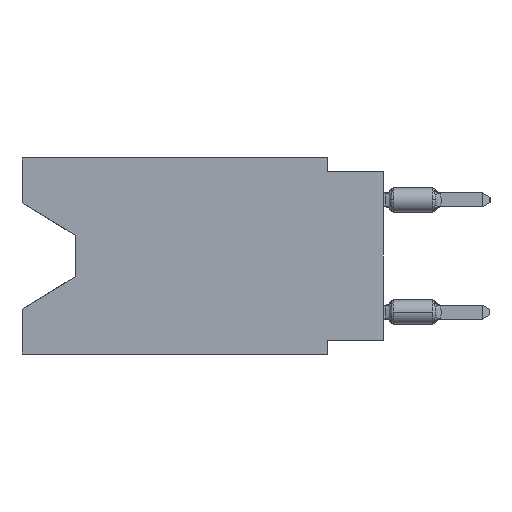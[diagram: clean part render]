
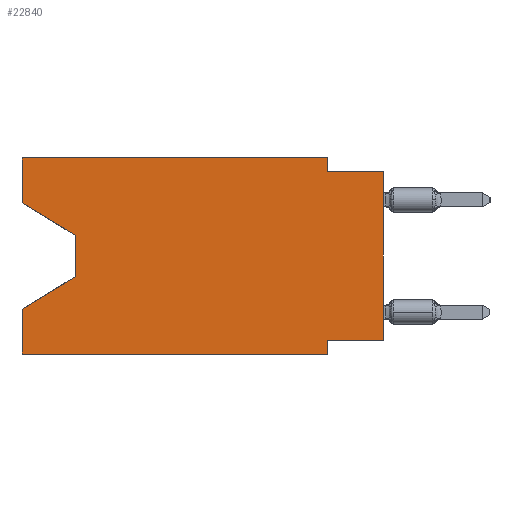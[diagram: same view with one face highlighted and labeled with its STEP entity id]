
A CAD part, left-side view. The second image highlights one B-rep face of the part: STEP entity #22840.
In plain terms, the highlighted planar face has unit normal (-1, 0, 0).
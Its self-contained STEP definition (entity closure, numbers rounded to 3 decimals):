
#190 = VERTEX_POINT ( 'NONE', #10890 ) ;
#904 = EDGE_LOOP ( 'NONE', ( #8589, #33899, #34542, #11193, #36317, #41280, #9095, #8226, #21461, #13554, #28977, #25182 ) ) ;
#2224 = LINE ( 'NONE', #29516, #17012 ) ;
#2622 = CARTESIAN_POINT ( 'NONE',  ( 0., 16.383, -2.038 ) ) ;
#5558 = EDGE_CURVE ( 'NONE', #40403, #23073, #16838, .T. ) ;
#5756 = CARTESIAN_POINT ( 'NONE',  ( 0., 16.383, -2.038 ) ) ;
#6208 = CARTESIAN_POINT ( 'NONE',  ( 0., 13.97, -5.385 ) ) ;
#6732 = CARTESIAN_POINT ( 'NONE',  ( 0., 13.97, -3.505 ) ) ;
#7610 = DIRECTION ( 'NONE',  ( 0., -1., 0. ) ) ;
#8206 = AXIS2_PLACEMENT_3D ( 'NONE', #37089, #36657, #29904 ) ;
#8226 = ORIENTED_EDGE ( 'NONE', *, *, #33989, .T. ) ;
#8589 = ORIENTED_EDGE ( 'NONE', *, *, #15736, .T. ) ;
#9095 = ORIENTED_EDGE ( 'NONE', *, *, #40701, .F. ) ;
#9105 = CARTESIAN_POINT ( 'NONE',  ( 0., 16.383, 0. ) ) ;
#9163 = CARTESIAN_POINT ( 'NONE',  ( 0., 2.54, -0.635 ) ) ;
#9471 = DIRECTION ( 'NONE',  ( 0., 0., 1. ) ) ;
#9561 = PLANE ( 'NONE',  #8206 ) ;
#9718 = VERTEX_POINT ( 'NONE', #30512 ) ;
#10890 = CARTESIAN_POINT ( 'NONE',  ( 0., 0., -8.255 ) ) ;
#11113 = LINE ( 'NONE', #13944, #34007 ) ;
#11193 = ORIENTED_EDGE ( 'NONE', *, *, #12792, .F. ) ;
#11499 = VECTOR ( 'NONE', #32435, 1000. ) ;
#12535 = LINE ( 'NONE', #39009, #38154 ) ;
#12792 = EDGE_CURVE ( 'NONE', #14418, #38018, #12535, .T. ) ;
#13004 = DIRECTION ( 'NONE',  ( 0., -1., 0. ) ) ;
#13524 = CARTESIAN_POINT ( 'NONE',  ( 0., 16.383, 0. ) ) ;
#13554 = ORIENTED_EDGE ( 'NONE', *, *, #5558, .F. ) ;
#13653 = EDGE_CURVE ( 'NONE', #9718, #40403, #20005, .T. ) ;
#13944 = CARTESIAN_POINT ( 'NONE',  ( 0., 13.97, -3.505 ) ) ;
#14418 = VERTEX_POINT ( 'NONE', #29110 ) ;
#14885 = EDGE_CURVE ( 'NONE', #36836, #35795, #22056, .T. ) ;
#14917 = VERTEX_POINT ( 'NONE', #2622 ) ;
#15736 = EDGE_CURVE ( 'NONE', #14917, #36433, #35714, .T. ) ;
#16089 = CARTESIAN_POINT ( 'NONE',  ( 0., 2.54, 0. ) ) ;
#16434 = CARTESIAN_POINT ( 'NONE',  ( 0., 2.54, -8.89 ) ) ;
#16674 = DIRECTION ( 'NONE',  ( 0., 0.855, -0.519 ) ) ;
#16838 = LINE ( 'NONE', #33683, #41931 ) ;
#17012 = VECTOR ( 'NONE', #29310, 1000. ) ;
#18340 = VECTOR ( 'NONE', #13004, 1000. ) ;
#18405 = EDGE_CURVE ( 'NONE', #39146, #38018, #36369, .T. ) ;
#19142 = CARTESIAN_POINT ( 'NONE',  ( 0., 16.383, -8.89 ) ) ;
#19164 = DIRECTION ( 'NONE',  ( 0., -1., 0. ) ) ;
#19407 = FACE_OUTER_BOUND ( 'NONE', #904, .T. ) ;
#20005 = LINE ( 'NONE', #9105, #21769 ) ;
#20494 = EDGE_CURVE ( 'NONE', #14418, #35795, #22855, .T. ) ;
#20990 = DIRECTION ( 'NONE',  ( 0., 0., -1. ) ) ;
#21461 = ORIENTED_EDGE ( 'NONE', *, *, #40191, .F. ) ;
#21604 = CARTESIAN_POINT ( 'NONE',  ( 0., 0., -0.635 ) ) ;
#21769 = VECTOR ( 'NONE', #19164, 1000. ) ;
#22056 = LINE ( 'NONE', #42412, #29543 ) ;
#22391 = DIRECTION ( 'NONE',  ( 0., 1., 0. ) ) ;
#22840 = ADVANCED_FACE ( 'NONE', ( #19407 ), #9561, .F. ) ;
#22855 = LINE ( 'NONE', #19142, #18340 ) ;
#23073 = VERTEX_POINT ( 'NONE', #9163 ) ;
#23202 = VECTOR ( 'NONE', #16674, 1000. ) ;
#23370 = LINE ( 'NONE', #13524, #30508 ) ;
#23520 = VECTOR ( 'NONE', #22391, 1000. ) ;
#24440 = DIRECTION ( 'NONE',  ( 0., 0., -1. ) ) ;
#25182 = ORIENTED_EDGE ( 'NONE', *, *, #32369, .F. ) ;
#25457 = CARTESIAN_POINT ( 'NONE',  ( 0., 0., -8.255 ) ) ;
#26019 = DIRECTION ( 'NONE',  ( 0., 0., 1. ) ) ;
#27126 = VERTEX_POINT ( 'NONE', #21604 ) ;
#28142 = LINE ( 'NONE', #41479, #33943 ) ;
#28838 = DIRECTION ( 'NONE',  ( 0., 0., -1. ) ) ;
#28949 = LINE ( 'NONE', #25457, #23520 ) ;
#28977 = ORIENTED_EDGE ( 'NONE', *, *, #13653, .F. ) ;
#29110 = CARTESIAN_POINT ( 'NONE',  ( 0., 16.383, -8.89 ) ) ;
#29310 = DIRECTION ( 'NONE',  ( 0., 0., 1. ) ) ;
#29516 = CARTESIAN_POINT ( 'NONE',  ( 0., 0., 0. ) ) ;
#29543 = VECTOR ( 'NONE', #28838, 1000. ) ;
#29904 = DIRECTION ( 'NONE',  ( 0., 0., -1. ) ) ;
#30508 = VECTOR ( 'NONE', #26019, 1000. ) ;
#30512 = CARTESIAN_POINT ( 'NONE',  ( 0., 16.383, 0. ) ) ;
#32369 = EDGE_CURVE ( 'NONE', #14917, #9718, #23370, .T. ) ;
#32435 = DIRECTION ( 'NONE',  ( 0., -0.855, -0.519 ) ) ;
#33683 = CARTESIAN_POINT ( 'NONE',  ( 0., 2.54, 0. ) ) ;
#33899 = ORIENTED_EDGE ( 'NONE', *, *, #43044, .T. ) ;
#33943 = VECTOR ( 'NONE', #7610, 1000. ) ;
#33989 = EDGE_CURVE ( 'NONE', #190, #27126, #2224, .T. ) ;
#34007 = VECTOR ( 'NONE', #24440, 1000. ) ;
#34542 = ORIENTED_EDGE ( 'NONE', *, *, #18405, .T. ) ;
#35714 = LINE ( 'NONE', #5756, #11499 ) ;
#35795 = VERTEX_POINT ( 'NONE', #16434 ) ;
#36317 = ORIENTED_EDGE ( 'NONE', *, *, #20494, .T. ) ;
#36369 = LINE ( 'NONE', #6208, #23202 ) ;
#36433 = VERTEX_POINT ( 'NONE', #6732 ) ;
#36657 = DIRECTION ( 'NONE',  ( 1., 0., 0. ) ) ;
#36836 = VERTEX_POINT ( 'NONE', #38417 ) ;
#37089 = CARTESIAN_POINT ( 'NONE',  ( 0., 16.383, 0. ) ) ;
#38018 = VERTEX_POINT ( 'NONE', #42358 ) ;
#38154 = VECTOR ( 'NONE', #9471, 1000. ) ;
#38417 = CARTESIAN_POINT ( 'NONE',  ( 0., 2.54, -8.255 ) ) ;
#39009 = CARTESIAN_POINT ( 'NONE',  ( 0., 16.383, 0. ) ) ;
#39146 = VERTEX_POINT ( 'NONE', #39270 ) ;
#39270 = CARTESIAN_POINT ( 'NONE',  ( 0., 13.97, -5.385 ) ) ;
#40191 = EDGE_CURVE ( 'NONE', #23073, #27126, #28142, .T. ) ;
#40403 = VERTEX_POINT ( 'NONE', #16089 ) ;
#40701 = EDGE_CURVE ( 'NONE', #190, #36836, #28949, .T. ) ;
#41280 = ORIENTED_EDGE ( 'NONE', *, *, #14885, .F. ) ;
#41479 = CARTESIAN_POINT ( 'NONE',  ( 0., 0., -0.635 ) ) ;
#41931 = VECTOR ( 'NONE', #20990, 1000. ) ;
#42358 = CARTESIAN_POINT ( 'NONE',  ( 0., 16.383, -6.852 ) ) ;
#42412 = CARTESIAN_POINT ( 'NONE',  ( 0., 2.54, -8.89 ) ) ;
#43044 = EDGE_CURVE ( 'NONE', #36433, #39146, #11113, .T. ) ;
